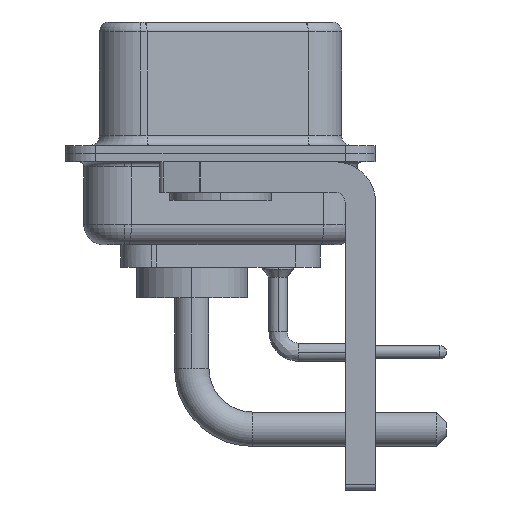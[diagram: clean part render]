
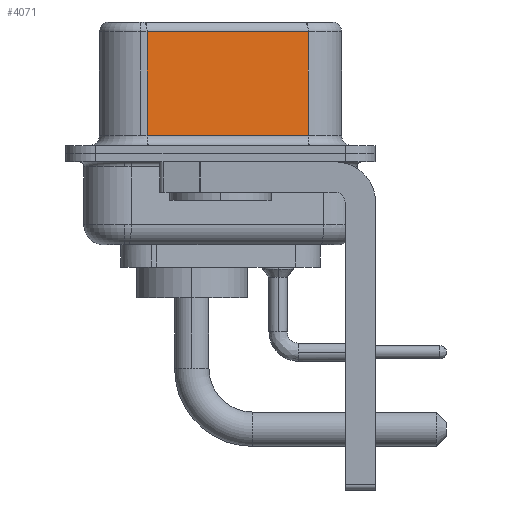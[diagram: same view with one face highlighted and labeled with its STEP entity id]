
A CAD part, left-side view. The second image highlights one B-rep face of the part: STEP entity #4071.
In plain terms, the highlighted planar face has unit normal (-0.985, -0.174, 0).
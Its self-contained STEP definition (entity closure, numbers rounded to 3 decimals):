
#230 = CARTESIAN_POINT ( 'NONE',  ( 3.73, 3.628, 6.02 ) ) ;
#919 = CARTESIAN_POINT ( 'NONE',  ( 5.132, -4.322, 6.52 ) ) ;
#1036 = VECTOR ( 'NONE', #4789, 1000. ) ;
#1044 = DIRECTION ( 'NONE',  ( 0., 0., -1. ) ) ;
#2019 = FACE_OUTER_BOUND ( 'NONE', #7646, .T. ) ;
#2257 = CARTESIAN_POINT ( 'NONE',  ( 3.73, 3.628, 0.9 ) ) ;
#3140 = EDGE_CURVE ( 'NONE', #11200, #20806, #20725, .T. ) ;
#3168 = LINE ( 'NONE', #919, #1036 ) ;
#3386 = VECTOR ( 'NONE', #6379, 1000. ) ;
#3930 = DIRECTION ( 'NONE',  ( -0.174, 0.985, 0. ) ) ;
#4071 = ADVANCED_FACE ( 'NONE', ( #2019 ), #15347, .F. ) ;
#4789 = DIRECTION ( 'NONE',  ( 0., 0., -1. ) ) ;
#5280 = ORIENTED_EDGE ( 'NONE', *, *, #22003, .T. ) ;
#5429 = EDGE_CURVE ( 'NONE', #18918, #17689, #8380, .T. ) ;
#6379 = DIRECTION ( 'NONE',  ( 0.174, -0.985, 0. ) ) ;
#7224 = ORIENTED_EDGE ( 'NONE', *, *, #14216, .F. ) ;
#7646 = EDGE_LOOP ( 'NONE', ( #7224, #12957, #5280, #12002 ) ) ;
#7983 = CARTESIAN_POINT ( 'NONE',  ( 5.132, -4.322, 6.02 ) ) ;
#8380 = LINE ( 'NONE', #23178, #3386 ) ;
#8525 = LINE ( 'NONE', #10390, #20535 ) ;
#9504 = CARTESIAN_POINT ( 'NONE',  ( 5.132, -4.322, 6.52 ) ) ;
#10390 = CARTESIAN_POINT ( 'NONE',  ( 3.73, 3.628, 6.52 ) ) ;
#11200 = VERTEX_POINT ( 'NONE', #7983 ) ;
#11762 = AXIS2_PLACEMENT_3D ( 'NONE', #9504, #13368, #13113 ) ;
#12002 = ORIENTED_EDGE ( 'NONE', *, *, #5429, .T. ) ;
#12957 = ORIENTED_EDGE ( 'NONE', *, *, #3140, .T. ) ;
#13113 = DIRECTION ( 'NONE',  ( -0.174, 0.985, 0. ) ) ;
#13251 = CARTESIAN_POINT ( 'NONE',  ( 5.132, -4.322, 6.02 ) ) ;
#13368 = DIRECTION ( 'NONE',  ( 0.985, 0.174, 0. ) ) ;
#14216 = EDGE_CURVE ( 'NONE', #11200, #17689, #3168, .T. ) ;
#15347 = PLANE ( 'NONE',  #11762 ) ;
#15854 = VECTOR ( 'NONE', #3930, 1000. ) ;
#17689 = VERTEX_POINT ( 'NONE', #23882 ) ;
#18918 = VERTEX_POINT ( 'NONE', #2257 ) ;
#20535 = VECTOR ( 'NONE', #1044, 1000. ) ;
#20725 = LINE ( 'NONE', #13251, #15854 ) ;
#20806 = VERTEX_POINT ( 'NONE', #230 ) ;
#22003 = EDGE_CURVE ( 'NONE', #20806, #18918, #8525, .T. ) ;
#23178 = CARTESIAN_POINT ( 'NONE',  ( 5.132, -4.322, 0.9 ) ) ;
#23882 = CARTESIAN_POINT ( 'NONE',  ( 5.132, -4.322, 0.9 ) ) ;
